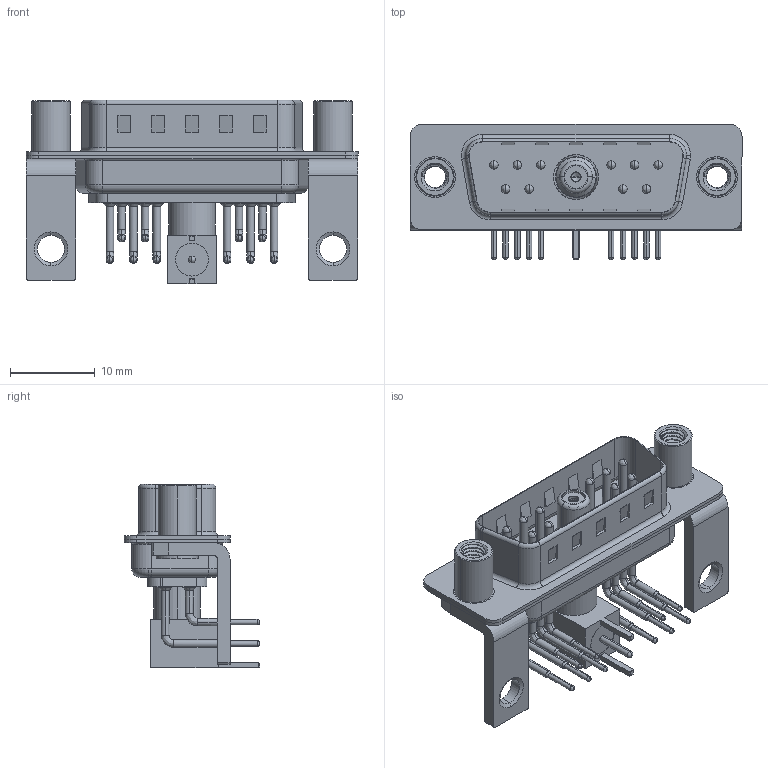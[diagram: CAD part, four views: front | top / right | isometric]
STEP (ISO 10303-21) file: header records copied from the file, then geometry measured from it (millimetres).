
FILE_DESCRIPTION (( 'STEP AP203' ), '1' );
FILE_NAME ('629-11W1240-7NE.STEP', '2022-05-09T20:00:28', ( '' ), ( '' ), 'SwSTEP 2.0', 'SolidWorks 2020', '' );
FILE_SCHEMA (( 'CONFIG_CONTROL_DESIGN' ));
Length unit declared in the file: millimetre
Products named in the file (16): 629Combo Contact Row 2; 629Combo Stabilizer Bracket; Socket_RA; RA Back Shell; 629Combo Contact Row 1; 629Combo Threaded Standoff_D; Insulator Socket; 629Combo Shell Rear_15 Contacts; Insulator RA Pin; Locking Collar; 629Combo Shell Front_15 Contacts; Co-Ax Jack_RA PC Tail; 629Combo Housing_11W1; Insulator Socket 2; Co-Ax Jack Assy_RA; 629-11W1240-7NE
Assembly tree (25 placements, depth 3):
  629-11W1240-7NE
    629Combo Housing_11W1
    629Combo Shell Rear_15 Contacts
    629Combo Shell Front_15 Contacts
    629Combo Stabilizer Bracket  x2
    629Combo Threaded Standoff_D  x2
    Co-Ax Jack Assy_RA
      Co-Ax Jack_RA PC Tail
      Insulator Socket
      Insulator Socket 2
      Locking Collar
      Socket_RA
      RA Back Shell
      Insulator RA Pin
    629Combo Contact Row 1  x6
    629Combo Contact Row 2  x4
Bounding box: 39.2 x 16 x 21.71 mm (x, y, z)
Volume: 2595.2 mm3; surface area: 7002.3 mm2
Topology: 24 solids, 27 shells, 1703 faces, 4605 edges, 2975 vertices
Faces by surface type: plane 867, cylinder 636, cone 75, bspline 67, torus 56, sphere 2
Entity records: 28728 total; most frequent: CARTESIAN_POINT 6926, DIRECTION 4301, ORIENTED_EDGE 4046, EDGE_CURVE 2023, AXIS2_PLACEMENT_3D 1568, VERTEX_POINT 1302, VECTOR 1165, LINE 1165
